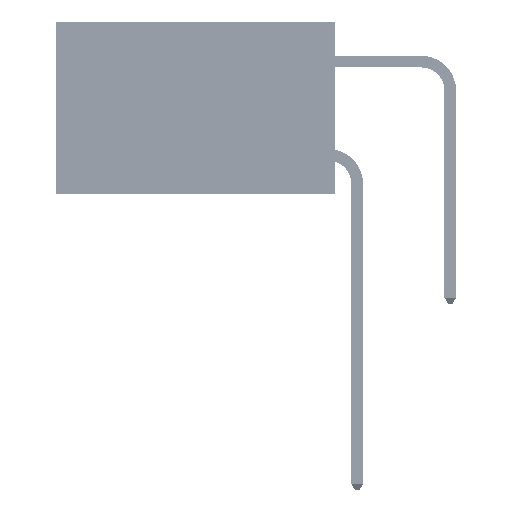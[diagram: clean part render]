
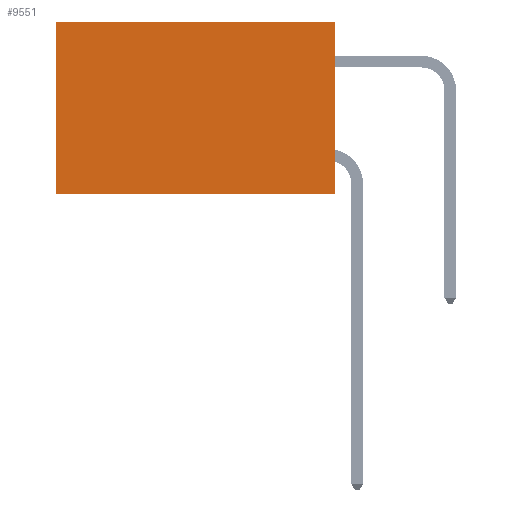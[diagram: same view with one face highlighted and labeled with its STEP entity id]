
A CAD part, left-side view. The second image highlights one B-rep face of the part: STEP entity #9551.
In plain terms, the highlighted planar face has unit normal (-1, 0, 0).
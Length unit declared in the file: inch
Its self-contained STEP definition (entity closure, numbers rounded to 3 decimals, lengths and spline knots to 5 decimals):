
#2299 = AXIS2_PLACEMENT_3D ( 'NONE', #29003, #32580, #25831 ) ;
#2700 = ORIENTED_EDGE ( 'NONE', *, *, #28194, .F. ) ;
#4352 = CARTESIAN_POINT ( 'NONE',  ( 0.2875, 0.6, -0.37 ) ) ;
#6055 = VECTOR ( 'NONE', #13089, 39.37008 ) ;
#7893 = VECTOR ( 'NONE', #15454, 39.37008 ) ;
#8499 = VECTOR ( 'NONE', #21702, 39.37008 ) ;
#9551 = ADVANCED_FACE ( 'NONE', ( #35183 ), #25360, .F. ) ;
#13033 = CARTESIAN_POINT ( 'NONE',  ( 0.2875, 0., 0. ) ) ;
#13089 = DIRECTION ( 'NONE',  ( 0., 0., -1. ) ) ;
#13293 = VERTEX_POINT ( 'NONE', #4352 ) ;
#15454 = DIRECTION ( 'NONE',  ( 0., 1., 0. ) ) ;
#16307 = CARTESIAN_POINT ( 'NONE',  ( 0.2875, 0., -0.37 ) ) ;
#18347 = EDGE_CURVE ( 'NONE', #37781, #13293, #24635, .T. ) ;
#19343 = ORIENTED_EDGE ( 'NONE', *, *, #18347, .T. ) ;
#21702 = DIRECTION ( 'NONE',  ( 0., 0., -1. ) ) ;
#22473 = DIRECTION ( 'NONE',  ( 0., 1., 0. ) ) ;
#23659 = VECTOR ( 'NONE', #22473, 39.37008 ) ;
#24635 = LINE ( 'NONE', #31506, #6055 ) ;
#24804 = ORIENTED_EDGE ( 'NONE', *, *, #44148, .F. ) ;
#25360 = PLANE ( 'NONE',  #2299 ) ;
#25492 = CARTESIAN_POINT ( 'NONE',  ( 0.2875, 0., 0. ) ) ;
#25831 = DIRECTION ( 'NONE',  ( 0., 0., -1. ) ) ;
#26829 = CARTESIAN_POINT ( 'NONE',  ( 0.2875, 0.6, 0. ) ) ;
#27675 = LINE ( 'NONE', #25492, #8499 ) ;
#28194 = EDGE_CURVE ( 'NONE', #40721, #28582, #27675, .T. ) ;
#28433 = EDGE_LOOP ( 'NONE', ( #19343, #24804, #2700, #30346 ) ) ;
#28582 = VERTEX_POINT ( 'NONE', #16307 ) ;
#29003 = CARTESIAN_POINT ( 'NONE',  ( 0.2875, 0., 0. ) ) ;
#29565 = CARTESIAN_POINT ( 'NONE',  ( 0.2875, 0., 0. ) ) ;
#30346 = ORIENTED_EDGE ( 'NONE', *, *, #39146, .T. ) ;
#31506 = CARTESIAN_POINT ( 'NONE',  ( 0.2875, 0.6, 0. ) ) ;
#32580 = DIRECTION ( 'NONE',  ( 1., 0., 0. ) ) ;
#33533 = CARTESIAN_POINT ( 'NONE',  ( 0.2875, 0., -0.37 ) ) ;
#35183 = FACE_OUTER_BOUND ( 'NONE', #28433, .T. ) ;
#36629 = LINE ( 'NONE', #29565, #23659 ) ;
#37155 = LINE ( 'NONE', #33533, #7893 ) ;
#37781 = VERTEX_POINT ( 'NONE', #26829 ) ;
#39146 = EDGE_CURVE ( 'NONE', #40721, #37781, #36629, .T. ) ;
#40721 = VERTEX_POINT ( 'NONE', #13033 ) ;
#44148 = EDGE_CURVE ( 'NONE', #28582, #13293, #37155, .T. ) ;
